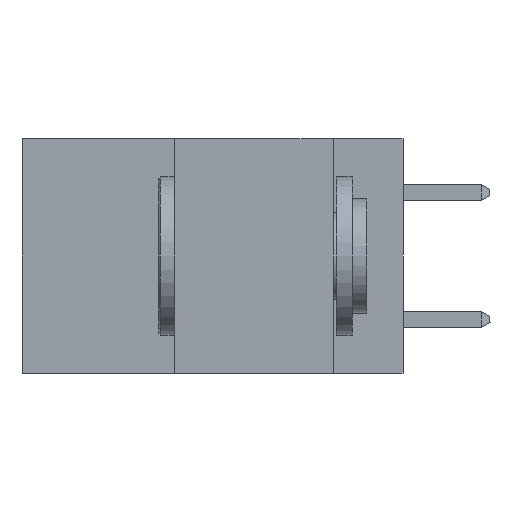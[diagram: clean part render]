
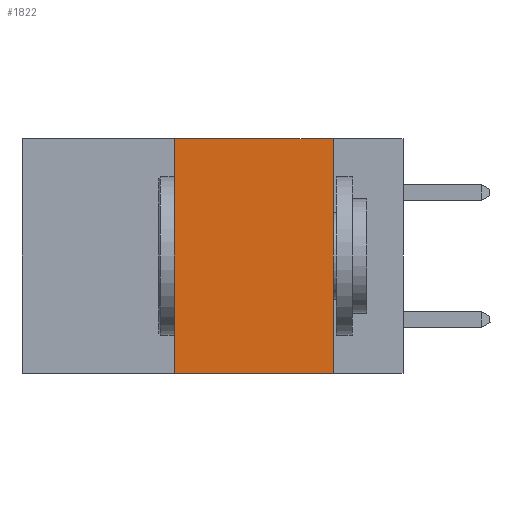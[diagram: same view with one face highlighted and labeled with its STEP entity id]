
A CAD part, left-side view. The second image highlights one B-rep face of the part: STEP entity #1822.
In plain terms, the highlighted planar face has unit normal (-1, 0, 0).
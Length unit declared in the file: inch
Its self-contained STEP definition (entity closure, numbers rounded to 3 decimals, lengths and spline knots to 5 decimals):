
#1822 = ADVANCED_FACE ( 'NONE', ( #15253 ), #31010, .F. ) ;
#3796 = ORIENTED_EDGE ( 'NONE', *, *, #40043, .F. ) ;
#7297 = CARTESIAN_POINT ( 'NONE',  ( 0., 0.11, -0.37 ) ) ;
#8087 = CARTESIAN_POINT ( 'NONE',  ( 0., 0.6, 0. ) ) ;
#8461 = ORIENTED_EDGE ( 'NONE', *, *, #41839, .T. ) ;
#8604 = VECTOR ( 'NONE', #31337, 39.37008 ) ;
#10637 = CARTESIAN_POINT ( 'NONE',  ( 0., 0.11, 0. ) ) ;
#10843 = CARTESIAN_POINT ( 'NONE',  ( 0., 0.36, 0. ) ) ;
#11238 = DIRECTION ( 'NONE',  ( 0., -1., 0. ) ) ;
#11516 = CARTESIAN_POINT ( 'NONE',  ( 0., 0.6, -0.37 ) ) ;
#14000 = VERTEX_POINT ( 'NONE', #27815 ) ;
#15253 = FACE_OUTER_BOUND ( 'NONE', #34583, .T. ) ;
#15340 = ORIENTED_EDGE ( 'NONE', *, *, #27081, .F. ) ;
#15968 = AXIS2_PLACEMENT_3D ( 'NONE', #8087, #31579, #34785 ) ;
#17159 = LINE ( 'NONE', #10843, #22429 ) ;
#18475 = LINE ( 'NONE', #11516, #28989 ) ;
#18698 = EDGE_CURVE ( 'NONE', #26746, #30469, #17159, .T. ) ;
#19387 = DIRECTION ( 'NONE',  ( 0., -1., 0. ) ) ;
#22429 = VECTOR ( 'NONE', #33885, 39.37008 ) ;
#22689 = CARTESIAN_POINT ( 'NONE',  ( 0., 0.36, -0.37 ) ) ;
#22783 = ORIENTED_EDGE ( 'NONE', *, *, #18698, .F. ) ;
#23366 = VECTOR ( 'NONE', #19387, 39.37008 ) ;
#26746 = VERTEX_POINT ( 'NONE', #22689 ) ;
#27081 = EDGE_CURVE ( 'NONE', #14000, #38336, #35372, .T. ) ;
#27815 = CARTESIAN_POINT ( 'NONE',  ( 0., 0.11, 0. ) ) ;
#28126 = LINE ( 'NONE', #39653, #23366 ) ;
#28989 = VECTOR ( 'NONE', #11238, 39.37008 ) ;
#30469 = VERTEX_POINT ( 'NONE', #38972 ) ;
#31010 = PLANE ( 'NONE',  #15968 ) ;
#31337 = DIRECTION ( 'NONE',  ( 0., 0., -1. ) ) ;
#31579 = DIRECTION ( 'NONE',  ( 1., 0., 0. ) ) ;
#33885 = DIRECTION ( 'NONE',  ( 0., 0., 1. ) ) ;
#34583 = EDGE_LOOP ( 'NONE', ( #15340, #3796, #22783, #8461 ) ) ;
#34785 = DIRECTION ( 'NONE',  ( 0., 0., -1. ) ) ;
#35372 = LINE ( 'NONE', #10637, #8604 ) ;
#38336 = VERTEX_POINT ( 'NONE', #7297 ) ;
#38972 = CARTESIAN_POINT ( 'NONE',  ( 0., 0.36, 0. ) ) ;
#39653 = CARTESIAN_POINT ( 'NONE',  ( 0., 0.6, 0. ) ) ;
#40043 = EDGE_CURVE ( 'NONE', #30469, #14000, #28126, .T. ) ;
#41839 = EDGE_CURVE ( 'NONE', #26746, #38336, #18475, .T. ) ;
